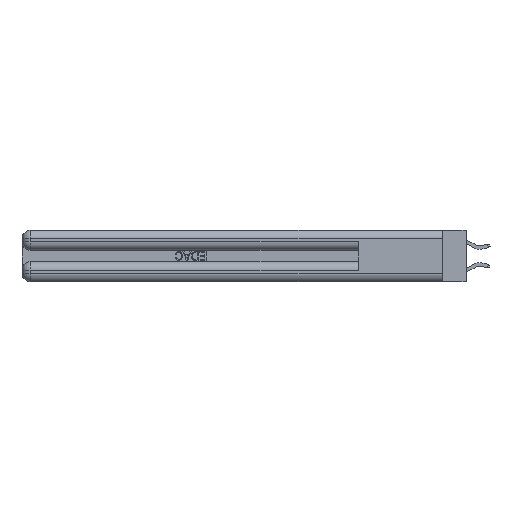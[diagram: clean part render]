
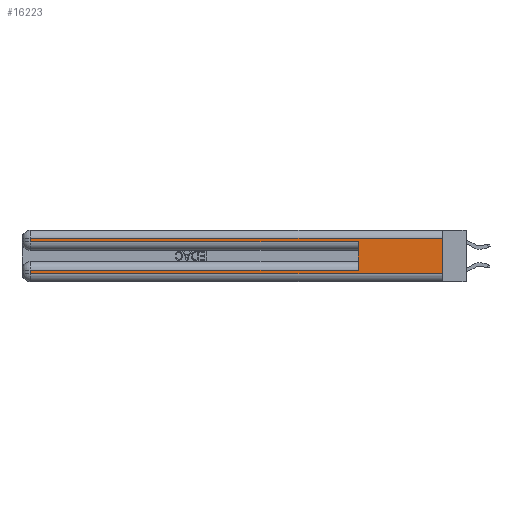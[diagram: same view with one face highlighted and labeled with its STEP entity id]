
A CAD part, left-side view. The second image highlights one B-rep face of the part: STEP entity #16223.
In plain terms, the highlighted planar face has unit normal (-1, 0, 0).
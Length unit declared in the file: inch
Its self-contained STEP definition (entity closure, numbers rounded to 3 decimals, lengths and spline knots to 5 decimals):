
#86 = DIRECTION ( 'NONE',  ( 0., 1., 0. ) ) ;
#899 = VECTOR ( 'NONE', #27775, 39.37008 ) ;
#2032 = VECTOR ( 'NONE', #32864, 39.37008 ) ;
#2658 = DIRECTION ( 'NONE',  ( 1., 0., 0. ) ) ;
#2762 = VECTOR ( 'NONE', #86, 39.37008 ) ;
#3279 = EDGE_CURVE ( 'NONE', #23571, #12091, #21049, .T. ) ;
#3291 = CARTESIAN_POINT ( 'NONE',  ( 0., 0., 0.06 ) ) ;
#3459 = VECTOR ( 'NONE', #33148, 39.37008 ) ;
#4274 = FACE_OUTER_BOUND ( 'NONE', #31134, .T. ) ;
#4705 = LINE ( 'NONE', #4736, #33861 ) ;
#4736 = CARTESIAN_POINT ( 'NONE',  ( 0., 0.6, 0.145 ) ) ;
#5113 = CARTESIAN_POINT ( 'NONE',  ( 0., 0., 0.285 ) ) ;
#5247 = CARTESIAN_POINT ( 'NONE',  ( 0., 2.94, 0.06 ) ) ;
#5956 = DIRECTION ( 'NONE',  ( 0., 0., -1. ) ) ;
#7412 = ORIENTED_EDGE ( 'NONE', *, *, #35059, .F. ) ;
#7773 = CARTESIAN_POINT ( 'NONE',  ( 0., 2.94, 0.31 ) ) ;
#8022 = AXIS2_PLACEMENT_3D ( 'NONE', #28038, #2658, #22488 ) ;
#8251 = EDGE_CURVE ( 'NONE', #9935, #27053, #36099, .T. ) ;
#8772 = VERTEX_POINT ( 'NONE', #29804 ) ;
#8991 = CARTESIAN_POINT ( 'NONE',  ( 0., 0., 0.31 ) ) ;
#9110 = EDGE_CURVE ( 'NONE', #21605, #23571, #32822, .T. ) ;
#9437 = CARTESIAN_POINT ( 'NONE',  ( 0., 0.6, 0.085 ) ) ;
#9935 = VERTEX_POINT ( 'NONE', #8991 ) ;
#10541 = CARTESIAN_POINT ( 'NONE',  ( 0., 0., 0.06 ) ) ;
#10699 = CARTESIAN_POINT ( 'NONE',  ( 0., 0., 0.37 ) ) ;
#11021 = LINE ( 'NONE', #30327, #3459 ) ;
#11565 = CARTESIAN_POINT ( 'NONE',  ( 0., 2.94, 0.37 ) ) ;
#12091 = VERTEX_POINT ( 'NONE', #5247 ) ;
#13552 = VECTOR ( 'NONE', #5956, 39.37008 ) ;
#13569 = DIRECTION ( 'NONE',  ( 0., 0., -1. ) ) ;
#14715 = DIRECTION ( 'NONE',  ( 0., -1., 0. ) ) ;
#15211 = ORIENTED_EDGE ( 'NONE', *, *, #23982, .T. ) ;
#16223 = ADVANCED_FACE ( 'NONE', ( #4274 ), #19657, .F. ) ;
#18037 = LINE ( 'NONE', #21556, #2032 ) ;
#19255 = ORIENTED_EDGE ( 'NONE', *, *, #24434, .T. ) ;
#19657 = PLANE ( 'NONE',  #8022 ) ;
#19927 = CARTESIAN_POINT ( 'NONE',  ( 0., 0., 0.085 ) ) ;
#21049 = LINE ( 'NONE', #11565, #13552 ) ;
#21126 = VECTOR ( 'NONE', #13569, 39.37008 ) ;
#21245 = EDGE_CURVE ( 'NONE', #9935, #30267, #11021, .T. ) ;
#21556 = CARTESIAN_POINT ( 'NONE',  ( 0., 2.94, 0.37 ) ) ;
#21605 = VERTEX_POINT ( 'NONE', #9437 ) ;
#21731 = DIRECTION ( 'NONE',  ( 0., 0., 1. ) ) ;
#22488 = DIRECTION ( 'NONE',  ( 0., 0., -1. ) ) ;
#23571 = VERTEX_POINT ( 'NONE', #34924 ) ;
#23982 = EDGE_CURVE ( 'NONE', #12091, #27053, #35863, .T. ) ;
#24054 = ORIENTED_EDGE ( 'NONE', *, *, #9110, .T. ) ;
#24434 = EDGE_CURVE ( 'NONE', #33225, #8772, #30979, .T. ) ;
#26971 = EDGE_CURVE ( 'NONE', #30267, #33225, #18037, .T. ) ;
#27053 = VERTEX_POINT ( 'NONE', #10541 ) ;
#27775 = DIRECTION ( 'NONE',  ( 0., -1., 0. ) ) ;
#28038 = CARTESIAN_POINT ( 'NONE',  ( 0., 0., 0.37 ) ) ;
#28377 = VECTOR ( 'NONE', #14715, 39.37008 ) ;
#29804 = CARTESIAN_POINT ( 'NONE',  ( 0., 0.6, 0.285 ) ) ;
#30267 = VERTEX_POINT ( 'NONE', #7773 ) ;
#30327 = CARTESIAN_POINT ( 'NONE',  ( 0., 0., 0.31 ) ) ;
#30979 = LINE ( 'NONE', #5113, #899 ) ;
#31134 = EDGE_LOOP ( 'NONE', ( #35301, #34799, #36258, #19255, #7412, #24054, #35029, #15211 ) ) ;
#32822 = LINE ( 'NONE', #19927, #2762 ) ;
#32864 = DIRECTION ( 'NONE',  ( 0., 0., -1. ) ) ;
#33148 = DIRECTION ( 'NONE',  ( 0., 1., 0. ) ) ;
#33225 = VERTEX_POINT ( 'NONE', #34630 ) ;
#33861 = VECTOR ( 'NONE', #21731, 39.37008 ) ;
#34630 = CARTESIAN_POINT ( 'NONE',  ( 0., 2.94, 0.285 ) ) ;
#34799 = ORIENTED_EDGE ( 'NONE', *, *, #21245, .T. ) ;
#34924 = CARTESIAN_POINT ( 'NONE',  ( 0., 2.94, 0.085 ) ) ;
#35029 = ORIENTED_EDGE ( 'NONE', *, *, #3279, .T. ) ;
#35059 = EDGE_CURVE ( 'NONE', #21605, #8772, #4705, .T. ) ;
#35301 = ORIENTED_EDGE ( 'NONE', *, *, #8251, .F. ) ;
#35863 = LINE ( 'NONE', #3291, #28377 ) ;
#36099 = LINE ( 'NONE', #10699, #21126 ) ;
#36258 = ORIENTED_EDGE ( 'NONE', *, *, #26971, .T. ) ;
